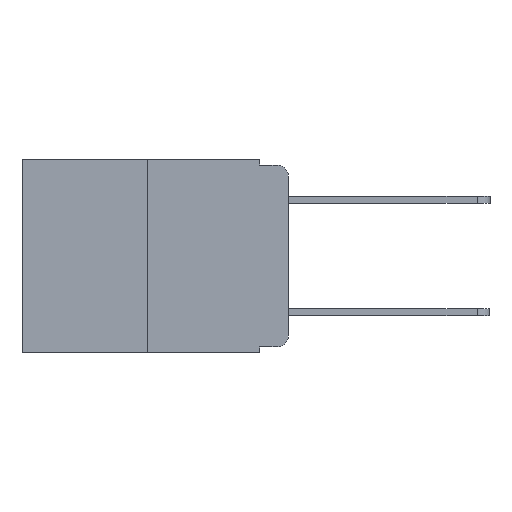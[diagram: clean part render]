
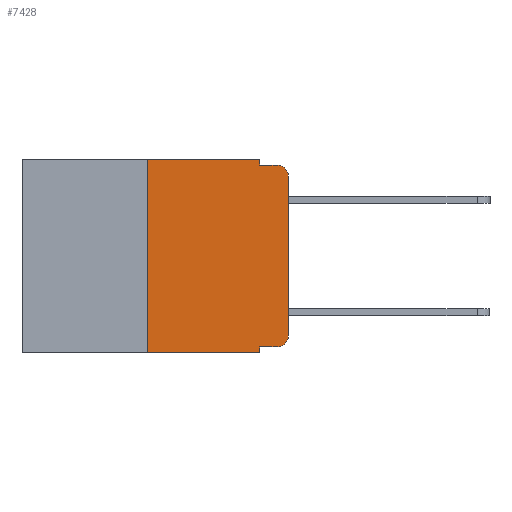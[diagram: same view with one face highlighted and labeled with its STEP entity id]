
A CAD part, left-side view. The second image highlights one B-rep face of the part: STEP entity #7428.
In plain terms, the highlighted planar face has unit normal (-1, 0, 0).
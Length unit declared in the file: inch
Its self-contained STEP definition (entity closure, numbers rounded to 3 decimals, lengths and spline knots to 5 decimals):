
#188 = EDGE_CURVE ( 'NONE', #1844, #8531, #10401, .T. ) ;
#301 = EDGE_CURVE ( 'NONE', #10394, #4474, #5202, .T. ) ;
#342 = EDGE_CURVE ( 'NONE', #4383, #6533, #7097, .T. ) ;
#425 = VERTEX_POINT ( 'NONE', #7670 ) ;
#560 = EDGE_CURVE ( 'NONE', #4383, #11896, #1730, .T. ) ;
#592 = EDGE_CURVE ( 'NONE', #11896, #1197, #9586, .T. ) ;
#1140 = DIRECTION ( 'NONE',  ( 1., 0., 0. ) ) ;
#1197 = VERTEX_POINT ( 'NONE', #11938 ) ;
#1580 = LINE ( 'NONE', #1678, #10112 ) ;
#1601 = EDGE_CURVE ( 'NONE', #4474, #1844, #11875, .T. ) ;
#1641 = CARTESIAN_POINT ( 'NONE',  ( 0., 0.02, -0.313 ) ) ;
#1678 = CARTESIAN_POINT ( 'NONE',  ( 0., 0.051, -0.01 ) ) ;
#1730 = LINE ( 'NONE', #8098, #12915 ) ;
#1844 = VERTEX_POINT ( 'NONE', #9005 ) ;
#1889 = CARTESIAN_POINT ( 'NONE',  ( 0., 0.02, -0.03 ) ) ;
#2213 = CARTESIAN_POINT ( 'NONE',  ( 0., 0.02, -0.01 ) ) ;
#2401 = AXIS2_PLACEMENT_3D ( 'NONE', #1641, #9474, #2829 ) ;
#2644 = ORIENTED_EDGE ( 'NONE', *, *, #11734, .T. ) ;
#2829 = DIRECTION ( 'NONE',  ( 0., 0., -1. ) ) ;
#2869 = DIRECTION ( 'NONE',  ( 0., -1., 0. ) ) ;
#2985 = CARTESIAN_POINT ( 'NONE',  ( 0., 0.051, 0. ) ) ;
#3032 = DIRECTION ( 'NONE',  ( 0., 0., -1. ) ) ;
#3420 = VECTOR ( 'NONE', #6473, 39.37008 ) ;
#4340 = LINE ( 'NONE', #12494, #13146 ) ;
#4383 = VERTEX_POINT ( 'NONE', #14239 ) ;
#4474 = VERTEX_POINT ( 'NONE', #6133 ) ;
#4755 = CARTESIAN_POINT ( 'NONE',  ( 0., 0.051, 0. ) ) ;
#4987 = ORIENTED_EDGE ( 'NONE', *, *, #6324, .T. ) ;
#5163 = ORIENTED_EDGE ( 'NONE', *, *, #560, .T. ) ;
#5174 = DIRECTION ( 'NONE',  ( 0., 0., 1. ) ) ;
#5202 = LINE ( 'NONE', #8477, #13255 ) ;
#5222 = FACE_OUTER_BOUND ( 'NONE', #9690, .T. ) ;
#5316 = AXIS2_PLACEMENT_3D ( 'NONE', #1889, #9655, #3032 ) ;
#5682 = CARTESIAN_POINT ( 'NONE',  ( 0., 0.25, -0.343 ) ) ;
#5828 = CARTESIAN_POINT ( 'NONE',  ( 0., 0.473, 0. ) ) ;
#5945 = DIRECTION ( 'NONE',  ( 0., -1., 0. ) ) ;
#6121 = AXIS2_PLACEMENT_3D ( 'NONE', #5828, #1140, #9108 ) ;
#6133 = CARTESIAN_POINT ( 'NONE',  ( 0., 0.25, 0. ) ) ;
#6168 = CIRCLE ( 'NONE', #5316, 0.02 ) ;
#6222 = DIRECTION ( 'NONE',  ( 0., 0., 1. ) ) ;
#6324 = EDGE_CURVE ( 'NONE', #10394, #6533, #13562, .T. ) ;
#6473 = DIRECTION ( 'NONE',  ( 0., -1., 0. ) ) ;
#6533 = VERTEX_POINT ( 'NONE', #11026 ) ;
#6815 = EDGE_CURVE ( 'NONE', #8531, #10119, #1580, .T. ) ;
#6966 = ORIENTED_EDGE ( 'NONE', *, *, #592, .T. ) ;
#7097 = LINE ( 'NONE', #2985, #12313 ) ;
#7189 = DIRECTION ( 'NONE',  ( 0., -1., 0. ) ) ;
#7428 = ADVANCED_FACE ( 'NONE', ( #5222 ), #8030, .F. ) ;
#7670 = CARTESIAN_POINT ( 'NONE',  ( 0., 0., -0.03 ) ) ;
#7672 = CARTESIAN_POINT ( 'NONE',  ( 0., 0.051, -0.01 ) ) ;
#8030 = PLANE ( 'NONE',  #6121 ) ;
#8098 = CARTESIAN_POINT ( 'NONE',  ( 0., 0.051, -0.333 ) ) ;
#8477 = CARTESIAN_POINT ( 'NONE',  ( 0., 0.25, 0. ) ) ;
#8531 = VERTEX_POINT ( 'NONE', #7672 ) ;
#8706 = ORIENTED_EDGE ( 'NONE', *, *, #188, .F. ) ;
#8830 = CARTESIAN_POINT ( 'NONE',  ( 0., 0.02, -0.333 ) ) ;
#9005 = CARTESIAN_POINT ( 'NONE',  ( 0., 0.051, 0. ) ) ;
#9108 = DIRECTION ( 'NONE',  ( 0., 0., -1. ) ) ;
#9474 = DIRECTION ( 'NONE',  ( -1., 0., 0. ) ) ;
#9586 = CIRCLE ( 'NONE', #2401, 0.02 ) ;
#9605 = ORIENTED_EDGE ( 'NONE', *, *, #1601, .F. ) ;
#9655 = DIRECTION ( 'NONE',  ( -1., 0., 0. ) ) ;
#9690 = EDGE_LOOP ( 'NONE', ( #13999, #2644, #14185, #8706, #9605, #9918, #4987, #13959, #5163, #6966 ) ) ;
#9918 = ORIENTED_EDGE ( 'NONE', *, *, #301, .F. ) ;
#10112 = VECTOR ( 'NONE', #2869, 39.37008 ) ;
#10119 = VERTEX_POINT ( 'NONE', #2213 ) ;
#10394 = VERTEX_POINT ( 'NONE', #5682 ) ;
#10401 = LINE ( 'NONE', #4755, #13097 ) ;
#11026 = CARTESIAN_POINT ( 'NONE',  ( 0., 0.051, -0.343 ) ) ;
#11190 = DIRECTION ( 'NONE',  ( 0., 0., -1. ) ) ;
#11710 = CARTESIAN_POINT ( 'NONE',  ( 0., 0.473, -0.343 ) ) ;
#11734 = EDGE_CURVE ( 'NONE', #425, #10119, #6168, .T. ) ;
#11875 = LINE ( 'NONE', #13385, #12196 ) ;
#11896 = VERTEX_POINT ( 'NONE', #8830 ) ;
#11938 = CARTESIAN_POINT ( 'NONE',  ( 0., 0., -0.313 ) ) ;
#12196 = VECTOR ( 'NONE', #7189, 39.37008 ) ;
#12313 = VECTOR ( 'NONE', #12646, 39.37008 ) ;
#12494 = CARTESIAN_POINT ( 'NONE',  ( 0., 0., 0. ) ) ;
#12646 = DIRECTION ( 'NONE',  ( 0., 0., -1. ) ) ;
#12915 = VECTOR ( 'NONE', #5945, 39.37008 ) ;
#12958 = EDGE_CURVE ( 'NONE', #1197, #425, #4340, .T. ) ;
#13097 = VECTOR ( 'NONE', #11190, 39.37008 ) ;
#13146 = VECTOR ( 'NONE', #6222, 39.37008 ) ;
#13255 = VECTOR ( 'NONE', #5174, 39.37008 ) ;
#13385 = CARTESIAN_POINT ( 'NONE',  ( 0., 0.473, 0. ) ) ;
#13562 = LINE ( 'NONE', #11710, #3420 ) ;
#13959 = ORIENTED_EDGE ( 'NONE', *, *, #342, .F. ) ;
#13999 = ORIENTED_EDGE ( 'NONE', *, *, #12958, .T. ) ;
#14185 = ORIENTED_EDGE ( 'NONE', *, *, #6815, .F. ) ;
#14239 = CARTESIAN_POINT ( 'NONE',  ( 0., 0.051, -0.333 ) ) ;
